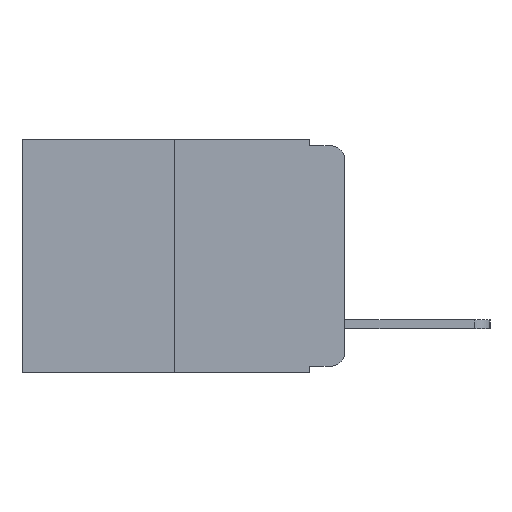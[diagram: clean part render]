
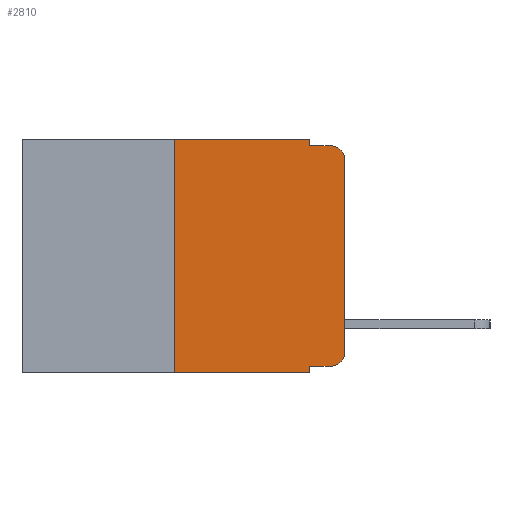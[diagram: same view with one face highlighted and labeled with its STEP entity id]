
A CAD part, left-side view. The second image highlights one B-rep face of the part: STEP entity #2810.
In plain terms, the highlighted planar face has unit normal (-1, 0, 0).
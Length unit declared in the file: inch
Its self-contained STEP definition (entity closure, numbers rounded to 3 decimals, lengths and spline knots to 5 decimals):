
#153 = ORIENTED_EDGE ( 'NONE', *, *, #6810, .T. ) ;
#443 = ORIENTED_EDGE ( 'NONE', *, *, #12532, .T. ) ;
#467 = ORIENTED_EDGE ( 'NONE', *, *, #11517, .F. ) ;
#556 = ORIENTED_EDGE ( 'NONE', *, *, #7420, .F. ) ;
#566 = DIRECTION ( 'NONE',  ( 0., -1., 0. ) ) ;
#768 = ORIENTED_EDGE ( 'NONE', *, *, #3187, .F. ) ;
#863 = VERTEX_POINT ( 'NONE', #1468 ) ;
#869 = ORIENTED_EDGE ( 'NONE', *, *, #9633, .T. ) ;
#1124 = VECTOR ( 'NONE', #13135, 39.37008 ) ;
#1296 = VECTOR ( 'NONE', #566, 39.37008 ) ;
#1468 = CARTESIAN_POINT ( 'NONE',  ( 0., 0.051, 0. ) ) ;
#1496 = CARTESIAN_POINT ( 'NONE',  ( 0., 0.473, 0. ) ) ;
#1568 = ORIENTED_EDGE ( 'NONE', *, *, #19994, .T. ) ;
#1634 = LINE ( 'NONE', #18656, #17591 ) ;
#2187 = ORIENTED_EDGE ( 'NONE', *, *, #6342, .F. ) ;
#2277 = ORIENTED_EDGE ( 'NONE', *, *, #8537, .F. ) ;
#2561 = VECTOR ( 'NONE', #17969, 39.37008 ) ;
#2721 = VECTOR ( 'NONE', #18352, 39.37008 ) ;
#2810 = ADVANCED_FACE ( 'NONE', ( #8953 ), #18497, .F. ) ;
#3051 = CARTESIAN_POINT ( 'NONE',  ( 0., 0.473, -0.343 ) ) ;
#3098 = CARTESIAN_POINT ( 'NONE',  ( 0., 0.051, -0.01 ) ) ;
#3187 = EDGE_CURVE ( 'NONE', #13419, #10769, #14887, .T. ) ;
#3341 = VERTEX_POINT ( 'NONE', #16845 ) ;
#3345 = VECTOR ( 'NONE', #8248, 39.37008 ) ;
#4030 = CIRCLE ( 'NONE', #12759, 0.02 ) ;
#4164 = AXIS2_PLACEMENT_3D ( 'NONE', #7368, #17998, #8918 ) ;
#5378 = LINE ( 'NONE', #11587, #1124 ) ;
#6342 = EDGE_CURVE ( 'NONE', #17198, #17921, #5378, .T. ) ;
#6548 = DIRECTION ( 'NONE',  ( 0., -1., 0. ) ) ;
#6590 = DIRECTION ( 'NONE',  ( 0., 0., -1. ) ) ;
#6767 = VERTEX_POINT ( 'NONE', #8035 ) ;
#6810 = EDGE_CURVE ( 'NONE', #7827, #7494, #1634, .T. ) ;
#7087 = VECTOR ( 'NONE', #6590, 39.37008 ) ;
#7337 = CARTESIAN_POINT ( 'NONE',  ( 0., 0.051, 0. ) ) ;
#7368 = CARTESIAN_POINT ( 'NONE',  ( 0., 0.02, -0.313 ) ) ;
#7420 = EDGE_CURVE ( 'NONE', #863, #18551, #18749, .T. ) ;
#7494 = VERTEX_POINT ( 'NONE', #14441 ) ;
#7784 = CARTESIAN_POINT ( 'NONE',  ( 0., 0.02, -0.03 ) ) ;
#7827 = VERTEX_POINT ( 'NONE', #15285 ) ;
#8035 = CARTESIAN_POINT ( 'NONE',  ( 0., 0.02, -0.333 ) ) ;
#8106 = DIRECTION ( 'NONE',  ( 0., 0., 1. ) ) ;
#8248 = DIRECTION ( 'NONE',  ( 0., -1., 0. ) ) ;
#8537 = EDGE_CURVE ( 'NONE', #17921, #863, #15064, .T. ) ;
#8917 = ORIENTED_EDGE ( 'NONE', *, *, #18997, .T. ) ;
#8918 = DIRECTION ( 'NONE',  ( 0., 0., -1. ) ) ;
#8953 = FACE_OUTER_BOUND ( 'NONE', #19085, .T. ) ;
#9113 = CARTESIAN_POINT ( 'NONE',  ( 0., 0.051, -0.333 ) ) ;
#9329 = DIRECTION ( 'NONE',  ( 0., 0., -1. ) ) ;
#9633 = EDGE_CURVE ( 'NONE', #17198, #10769, #15047, .T. ) ;
#10769 = VERTEX_POINT ( 'NONE', #13940 ) ;
#10937 = DIRECTION ( 'NONE',  ( 0., 0., -1. ) ) ;
#10996 = VECTOR ( 'NONE', #6548, 39.37008 ) ;
#11517 = EDGE_CURVE ( 'NONE', #18551, #3341, #19648, .T. ) ;
#11587 = CARTESIAN_POINT ( 'NONE',  ( 0., 0.25, 0. ) ) ;
#11604 = CARTESIAN_POINT ( 'NONE',  ( 0., 0.051, -0.333 ) ) ;
#12532 = EDGE_CURVE ( 'NONE', #7494, #3341, #4030, .T. ) ;
#12542 = CARTESIAN_POINT ( 'NONE',  ( 0., 0.25, -0.343 ) ) ;
#12759 = AXIS2_PLACEMENT_3D ( 'NONE', #7784, #18402, #9329 ) ;
#13135 = DIRECTION ( 'NONE',  ( 0., 0., 1. ) ) ;
#13419 = VERTEX_POINT ( 'NONE', #9113 ) ;
#13940 = CARTESIAN_POINT ( 'NONE',  ( 0., 0.051, -0.343 ) ) ;
#14441 = CARTESIAN_POINT ( 'NONE',  ( 0., 0., -0.03 ) ) ;
#14887 = LINE ( 'NONE', #7337, #2561 ) ;
#15047 = LINE ( 'NONE', #3051, #2721 ) ;
#15064 = LINE ( 'NONE', #15722, #10996 ) ;
#15285 = CARTESIAN_POINT ( 'NONE',  ( 0., 0., -0.313 ) ) ;
#15722 = CARTESIAN_POINT ( 'NONE',  ( 0., 0.473, 0. ) ) ;
#15843 = CARTESIAN_POINT ( 'NONE',  ( 0., 0.25, 0. ) ) ;
#16845 = CARTESIAN_POINT ( 'NONE',  ( 0., 0.02, -0.01 ) ) ;
#17198 = VERTEX_POINT ( 'NONE', #12542 ) ;
#17591 = VECTOR ( 'NONE', #8106, 39.37008 ) ;
#17921 = VERTEX_POINT ( 'NONE', #15843 ) ;
#17969 = DIRECTION ( 'NONE',  ( 0., 0., -1. ) ) ;
#17998 = DIRECTION ( 'NONE',  ( -1., 0., 0. ) ) ;
#18097 = AXIS2_PLACEMENT_3D ( 'NONE', #1496, #20008, #10937 ) ;
#18226 = LINE ( 'NONE', #11604, #1296 ) ;
#18352 = DIRECTION ( 'NONE',  ( 0., -1., 0. ) ) ;
#18402 = DIRECTION ( 'NONE',  ( -1., 0., 0. ) ) ;
#18497 = PLANE ( 'NONE',  #18097 ) ;
#18551 = VERTEX_POINT ( 'NONE', #3098 ) ;
#18656 = CARTESIAN_POINT ( 'NONE',  ( 0., 0., 0. ) ) ;
#18749 = LINE ( 'NONE', #18797, #7087 ) ;
#18794 = CARTESIAN_POINT ( 'NONE',  ( 0., 0.051, -0.01 ) ) ;
#18797 = CARTESIAN_POINT ( 'NONE',  ( 0., 0.051, 0. ) ) ;
#18991 = CIRCLE ( 'NONE', #4164, 0.02 ) ;
#18997 = EDGE_CURVE ( 'NONE', #6767, #7827, #18991, .T. ) ;
#19085 = EDGE_LOOP ( 'NONE', ( #153, #443, #467, #556, #2277, #2187, #869, #768, #1568, #8917 ) ) ;
#19648 = LINE ( 'NONE', #18794, #3345 ) ;
#19994 = EDGE_CURVE ( 'NONE', #13419, #6767, #18226, .T. ) ;
#20008 = DIRECTION ( 'NONE',  ( 1., 0., 0. ) ) ;
